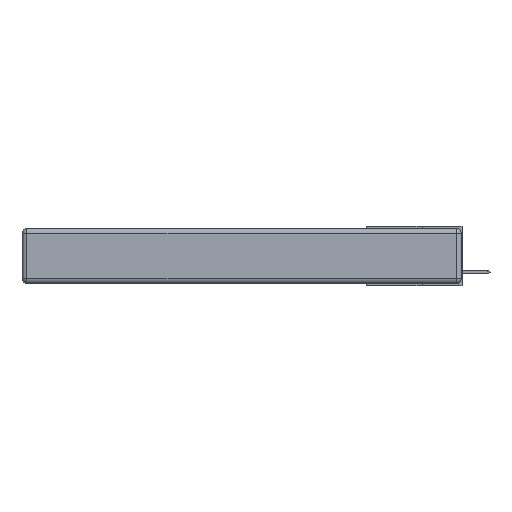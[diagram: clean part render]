
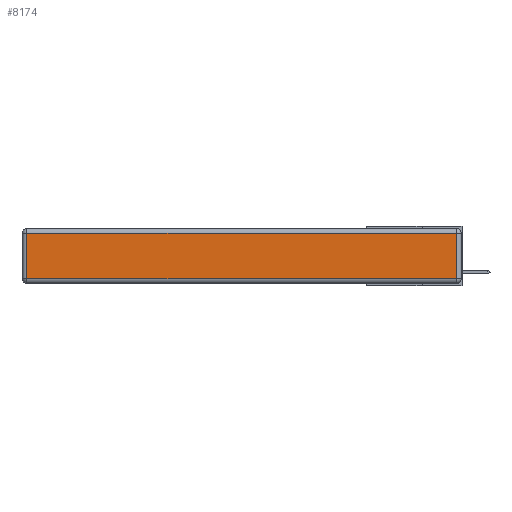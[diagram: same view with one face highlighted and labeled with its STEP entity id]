
A CAD part, left-side view. The second image highlights one B-rep face of the part: STEP entity #8174.
In plain terms, the highlighted planar face has unit normal (-1, 0, 0).
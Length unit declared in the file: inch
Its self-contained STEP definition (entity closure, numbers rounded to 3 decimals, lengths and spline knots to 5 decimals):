
#3 = CARTESIAN_POINT ( 'NONE',  ( 0., 0., -0.313 ) ) ;
#419 = LINE ( 'NONE', #3, #11025 ) ;
#480 = LINE ( 'NONE', #10564, #11622 ) ;
#580 = ORIENTED_EDGE ( 'NONE', *, *, #12026, .T. ) ;
#742 = AXIS2_PLACEMENT_3D ( 'NONE', #2592, #6138, #6034 ) ;
#1576 = PLANE ( 'NONE',  #742 ) ;
#2592 = CARTESIAN_POINT ( 'NONE',  ( 0., 0., -0.343 ) ) ;
#3480 = VECTOR ( 'NONE', #9320, 39.37008 ) ;
#3700 = CARTESIAN_POINT ( 'NONE',  ( 0., 2.72, -0.313 ) ) ;
#4001 = LINE ( 'NONE', #13809, #3480 ) ;
#4211 = VERTEX_POINT ( 'NONE', #12290 ) ;
#4384 = ORIENTED_EDGE ( 'NONE', *, *, #14423, .T. ) ;
#5061 = VERTEX_POINT ( 'NONE', #3700 ) ;
#5392 = VERTEX_POINT ( 'NONE', #12581 ) ;
#5697 = CARTESIAN_POINT ( 'NONE',  ( 0., 0.03, -0.03 ) ) ;
#6034 = DIRECTION ( 'NONE',  ( 0., 0., 1. ) ) ;
#6138 = DIRECTION ( 'NONE',  ( -1., 0., 0. ) ) ;
#6414 = EDGE_CURVE ( 'NONE', #10310, #5392, #480, .T. ) ;
#6531 = FACE_OUTER_BOUND ( 'NONE', #7899, .T. ) ;
#7678 = CARTESIAN_POINT ( 'NONE',  ( 0., 0.03, -0.343 ) ) ;
#7899 = EDGE_LOOP ( 'NONE', ( #580, #4384, #14274, #8551 ) ) ;
#8174 = ADVANCED_FACE ( 'NONE', ( #6531 ), #1576, .T. ) ;
#8551 = ORIENTED_EDGE ( 'NONE', *, *, #11005, .T. ) ;
#9320 = DIRECTION ( 'NONE',  ( 0., 0., -1. ) ) ;
#9901 = LINE ( 'NONE', #7678, #12524 ) ;
#10310 = VERTEX_POINT ( 'NONE', #5697 ) ;
#10564 = CARTESIAN_POINT ( 'NONE',  ( 0., 2.75, -0.03 ) ) ;
#11005 = EDGE_CURVE ( 'NONE', #5392, #5061, #4001, .T. ) ;
#11025 = VECTOR ( 'NONE', #14256, 39.37008 ) ;
#11622 = VECTOR ( 'NONE', #11648, 39.37008 ) ;
#11648 = DIRECTION ( 'NONE',  ( 0., 1., 0. ) ) ;
#12026 = EDGE_CURVE ( 'NONE', #5061, #4211, #419, .T. ) ;
#12290 = CARTESIAN_POINT ( 'NONE',  ( 0., 0.03, -0.313 ) ) ;
#12524 = VECTOR ( 'NONE', #13129, 39.37008 ) ;
#12581 = CARTESIAN_POINT ( 'NONE',  ( 0., 2.72, -0.03 ) ) ;
#13129 = DIRECTION ( 'NONE',  ( 0., 0., 1. ) ) ;
#13809 = CARTESIAN_POINT ( 'NONE',  ( 0., 2.72, -0.343 ) ) ;
#14256 = DIRECTION ( 'NONE',  ( 0., -1., 0. ) ) ;
#14274 = ORIENTED_EDGE ( 'NONE', *, *, #6414, .T. ) ;
#14423 = EDGE_CURVE ( 'NONE', #4211, #10310, #9901, .T. ) ;
